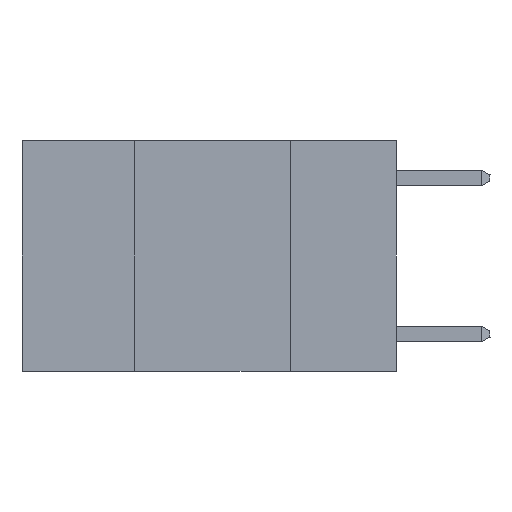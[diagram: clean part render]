
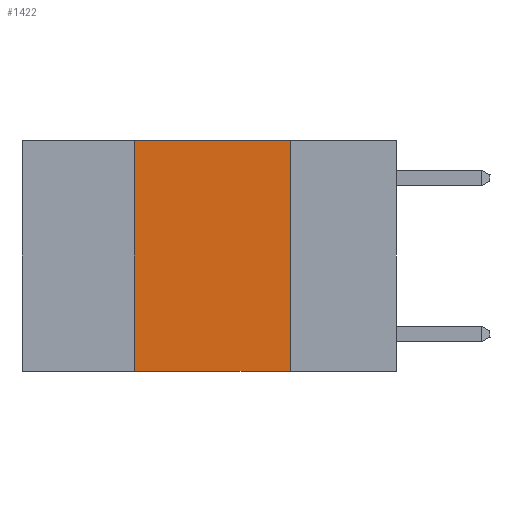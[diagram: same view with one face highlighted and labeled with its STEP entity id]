
A CAD part, left-side view. The second image highlights one B-rep face of the part: STEP entity #1422.
In plain terms, the highlighted planar face has unit normal (-1, 0, 0).
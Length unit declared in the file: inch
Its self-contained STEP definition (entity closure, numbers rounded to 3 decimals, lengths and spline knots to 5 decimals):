
#1206 = ORIENTED_EDGE ( 'NONE', *, *, #1946, .T. ) ;
#1422 = ADVANCED_FACE ( 'NONE', ( #10361 ), #8459, .F. ) ;
#1905 = VERTEX_POINT ( 'NONE', #18312 ) ;
#1946 = EDGE_CURVE ( 'NONE', #16971, #20346, #11940, .T. ) ;
#2407 = CARTESIAN_POINT ( 'NONE',  ( 0., 0.6, 0. ) ) ;
#3053 = ORIENTED_EDGE ( 'NONE', *, *, #9554, .F. ) ;
#3775 = CARTESIAN_POINT ( 'NONE',  ( 0., 0.6, -0.37 ) ) ;
#4316 = ORIENTED_EDGE ( 'NONE', *, *, #17169, .F. ) ;
#4338 = CARTESIAN_POINT ( 'NONE',  ( 0., 0.17, 0. ) ) ;
#5466 = CARTESIAN_POINT ( 'NONE',  ( 0., 0.6, 0. ) ) ;
#6382 = CARTESIAN_POINT ( 'NONE',  ( 0., 0.42, 0. ) ) ;
#7575 = VECTOR ( 'NONE', #16598, 39.37008 ) ;
#8459 = PLANE ( 'NONE',  #12133 ) ;
#8602 = VECTOR ( 'NONE', #12408, 39.37008 ) ;
#8672 = CARTESIAN_POINT ( 'NONE',  ( 0., 0.17, -0.37 ) ) ;
#8769 = DIRECTION ( 'NONE',  ( 1., 0., 0. ) ) ;
#9554 = EDGE_CURVE ( 'NONE', #16517, #20346, #20632, .T. ) ;
#9817 = LINE ( 'NONE', #6382, #16714 ) ;
#9924 = DIRECTION ( 'NONE',  ( 0., 0., 1. ) ) ;
#10110 = EDGE_CURVE ( 'NONE', #16971, #1905, #9817, .T. ) ;
#10361 = FACE_OUTER_BOUND ( 'NONE', #15793, .T. ) ;
#10634 = ORIENTED_EDGE ( 'NONE', *, *, #10110, .F. ) ;
#11849 = DIRECTION ( 'NONE',  ( 0., 0., -1. ) ) ;
#11868 = LINE ( 'NONE', #5466, #7575 ) ;
#11940 = LINE ( 'NONE', #3775, #16448 ) ;
#12133 = AXIS2_PLACEMENT_3D ( 'NONE', #2407, #8769, #11849 ) ;
#12408 = DIRECTION ( 'NONE',  ( 0., 0., -1. ) ) ;
#14838 = CARTESIAN_POINT ( 'NONE',  ( 0., 0.17, 0. ) ) ;
#15793 = EDGE_LOOP ( 'NONE', ( #3053, #4316, #10634, #1206 ) ) ;
#16448 = VECTOR ( 'NONE', #18058, 39.37008 ) ;
#16517 = VERTEX_POINT ( 'NONE', #14838 ) ;
#16598 = DIRECTION ( 'NONE',  ( 0., -1., 0. ) ) ;
#16714 = VECTOR ( 'NONE', #9924, 39.37008 ) ;
#16971 = VERTEX_POINT ( 'NONE', #19343 ) ;
#17169 = EDGE_CURVE ( 'NONE', #1905, #16517, #11868, .T. ) ;
#18058 = DIRECTION ( 'NONE',  ( 0., -1., 0. ) ) ;
#18312 = CARTESIAN_POINT ( 'NONE',  ( 0., 0.42, 0. ) ) ;
#19343 = CARTESIAN_POINT ( 'NONE',  ( 0., 0.42, -0.37 ) ) ;
#20346 = VERTEX_POINT ( 'NONE', #8672 ) ;
#20632 = LINE ( 'NONE', #4338, #8602 ) ;
